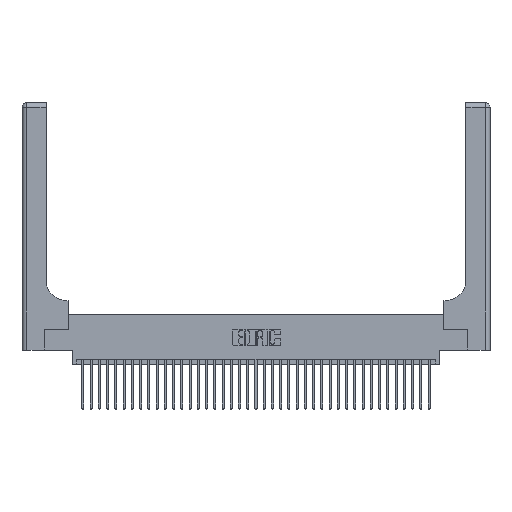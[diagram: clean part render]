
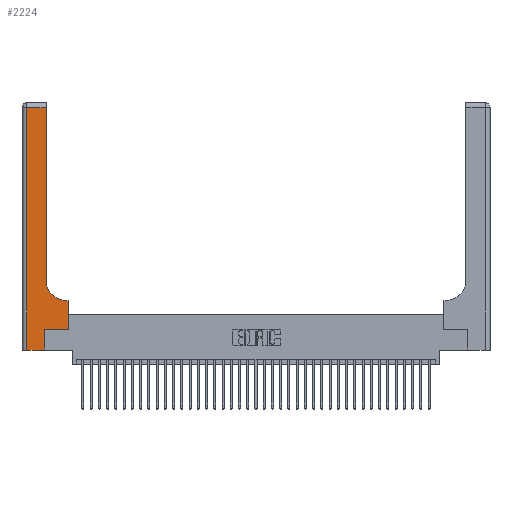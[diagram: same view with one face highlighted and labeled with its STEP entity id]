
A CAD part, top view. The second image highlights one B-rep face of the part: STEP entity #2224.
In plain terms, the highlighted planar face has unit normal (0, 0, 1).
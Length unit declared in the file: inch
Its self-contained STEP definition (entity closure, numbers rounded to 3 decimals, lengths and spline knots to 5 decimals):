
#657 = CARTESIAN_POINT ( 'NONE',  ( 0., 2.94, 0.37 ) ) ;
#1552 = CARTESIAN_POINT ( 'NONE',  ( 0., 3., 0.37 ) ) ;
#1670 = VECTOR ( 'NONE', #33518, 39.37008 ) ;
#2224 = ADVANCED_FACE ( 'NONE', ( #31966 ), #31536, .F. ) ;
#2609 = VERTEX_POINT ( 'NONE', #21635 ) ;
#2968 = EDGE_LOOP ( 'NONE', ( #31132, #36995, #37355, #5394, #27373, #5549, #32895, #32816, #12002 ) ) ;
#3416 = EDGE_CURVE ( 'NONE', #30023, #18984, #8344, .T. ) ;
#3952 = CARTESIAN_POINT ( 'NONE',  ( 0.2915, 2.94, 0.37 ) ) ;
#4515 = CARTESIAN_POINT ( 'NONE',  ( 0.5585, 0.25, 0.37 ) ) ;
#4913 = VERTEX_POINT ( 'NONE', #22307 ) ;
#5001 = LINE ( 'NONE', #31647, #20967 ) ;
#5394 = ORIENTED_EDGE ( 'NONE', *, *, #19630, .T. ) ;
#5549 = ORIENTED_EDGE ( 'NONE', *, *, #12118, .T. ) ;
#5668 = CARTESIAN_POINT ( 'NONE',  ( 0.269, 0., 0.37 ) ) ;
#5989 = DIRECTION ( 'NONE',  ( 0., 0., -1. ) ) ;
#6431 = CARTESIAN_POINT ( 'NONE',  ( 0.269, 0., 0.37 ) ) ;
#7412 = VECTOR ( 'NONE', #22506, 39.37008 ) ;
#8344 = LINE ( 'NONE', #4515, #7412 ) ;
#8436 = VERTEX_POINT ( 'NONE', #5668 ) ;
#8699 = DIRECTION ( 'NONE',  ( 0., -1., 0. ) ) ;
#9133 = VECTOR ( 'NONE', #8699, 39.37008 ) ;
#9220 = CIRCLE ( 'NONE', #18550, 0.25 ) ;
#9683 = LINE ( 'NONE', #6431, #1670 ) ;
#10200 = LINE ( 'NONE', #657, #26183 ) ;
#10659 = DIRECTION ( 'NONE',  ( 0., 0., -1. ) ) ;
#12002 = ORIENTED_EDGE ( 'NONE', *, *, #31974, .T. ) ;
#12118 = EDGE_CURVE ( 'NONE', #15676, #30023, #12529, .T. ) ;
#12529 = LINE ( 'NONE', #30538, #19614 ) ;
#13780 = EDGE_CURVE ( 'NONE', #4913, #22943, #34080, .T. ) ;
#13802 = DIRECTION ( 'NONE',  ( 1., 0., 0. ) ) ;
#13936 = CARTESIAN_POINT ( 'NONE',  ( 0., 0., 0.37 ) ) ;
#13968 = CARTESIAN_POINT ( 'NONE',  ( 0.5585, 0.6, 0.37 ) ) ;
#14592 = CARTESIAN_POINT ( 'NONE',  ( 0.2915, 0.85, 0.37 ) ) ;
#15303 = LINE ( 'NONE', #13936, #31288 ) ;
#15444 = DIRECTION ( 'NONE',  ( 1., 0., 0. ) ) ;
#15676 = VERTEX_POINT ( 'NONE', #26804 ) ;
#17661 = CARTESIAN_POINT ( 'NONE',  ( 0.06, 3., 0.37 ) ) ;
#18550 = AXIS2_PLACEMENT_3D ( 'NONE', #23989, #5989, #26993 ) ;
#18984 = VERTEX_POINT ( 'NONE', #13968 ) ;
#19310 = EDGE_CURVE ( 'NONE', #8436, #15676, #9683, .T. ) ;
#19614 = VECTOR ( 'NONE', #15444, 39.37008 ) ;
#19630 = EDGE_CURVE ( 'NONE', #22943, #8436, #15303, .T. ) ;
#19736 = DIRECTION ( 'NONE',  ( 0., 1., 0. ) ) ;
#19742 = DIRECTION ( 'NONE',  ( -1., 0., 0. ) ) ;
#20540 = EDGE_CURVE ( 'NONE', #27932, #4913, #10200, .T. ) ;
#20967 = VECTOR ( 'NONE', #19742, 39.37008 ) ;
#21635 = CARTESIAN_POINT ( 'NONE',  ( 0.5415, 0.6, 0.37 ) ) ;
#22307 = CARTESIAN_POINT ( 'NONE',  ( 0.06, 2.94, 0.37 ) ) ;
#22506 = DIRECTION ( 'NONE',  ( 0., 1., 0. ) ) ;
#22943 = VERTEX_POINT ( 'NONE', #32957 ) ;
#23019 = LINE ( 'NONE', #31776, #38962 ) ;
#23989 = CARTESIAN_POINT ( 'NONE',  ( 0.5415, 0.85, 0.37 ) ) ;
#26183 = VECTOR ( 'NONE', #30790, 39.37008 ) ;
#26804 = CARTESIAN_POINT ( 'NONE',  ( 0.269, 0.25, 0.37 ) ) ;
#26993 = DIRECTION ( 'NONE',  ( 1., 0., 0. ) ) ;
#27373 = ORIENTED_EDGE ( 'NONE', *, *, #19310, .T. ) ;
#27932 = VERTEX_POINT ( 'NONE', #3952 ) ;
#29907 = EDGE_CURVE ( 'NONE', #35274, #27932, #23019, .T. ) ;
#29929 = AXIS2_PLACEMENT_3D ( 'NONE', #1552, #10659, #31664 ) ;
#30023 = VERTEX_POINT ( 'NONE', #35432 ) ;
#30538 = CARTESIAN_POINT ( 'NONE',  ( 0.269, 0.25, 0.37 ) ) ;
#30790 = DIRECTION ( 'NONE',  ( -1., 0., 0. ) ) ;
#31132 = ORIENTED_EDGE ( 'NONE', *, *, #29907, .T. ) ;
#31288 = VECTOR ( 'NONE', #13802, 39.37008 ) ;
#31536 = PLANE ( 'NONE',  #29929 ) ;
#31647 = CARTESIAN_POINT ( 'NONE',  ( 0.2915, 0.6, 0.37 ) ) ;
#31664 = DIRECTION ( 'NONE',  ( -1., 0., 0. ) ) ;
#31776 = CARTESIAN_POINT ( 'NONE',  ( 0.2915, 3., 0.37 ) ) ;
#31966 = FACE_OUTER_BOUND ( 'NONE', #2968, .T. ) ;
#31974 = EDGE_CURVE ( 'NONE', #2609, #35274, #9220, .T. ) ;
#32816 = ORIENTED_EDGE ( 'NONE', *, *, #33502, .T. ) ;
#32895 = ORIENTED_EDGE ( 'NONE', *, *, #3416, .T. ) ;
#32957 = CARTESIAN_POINT ( 'NONE',  ( 0.06, 0., 0.37 ) ) ;
#33502 = EDGE_CURVE ( 'NONE', #18984, #2609, #5001, .T. ) ;
#33518 = DIRECTION ( 'NONE',  ( 0., 1., 0. ) ) ;
#34080 = LINE ( 'NONE', #17661, #9133 ) ;
#35274 = VERTEX_POINT ( 'NONE', #14592 ) ;
#35432 = CARTESIAN_POINT ( 'NONE',  ( 0.5585, 0.25, 0.37 ) ) ;
#36995 = ORIENTED_EDGE ( 'NONE', *, *, #20540, .T. ) ;
#37355 = ORIENTED_EDGE ( 'NONE', *, *, #13780, .T. ) ;
#38962 = VECTOR ( 'NONE', #19736, 39.37008 ) ;
